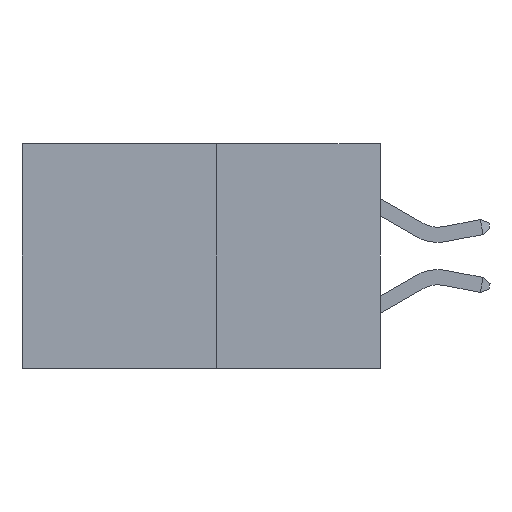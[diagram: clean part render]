
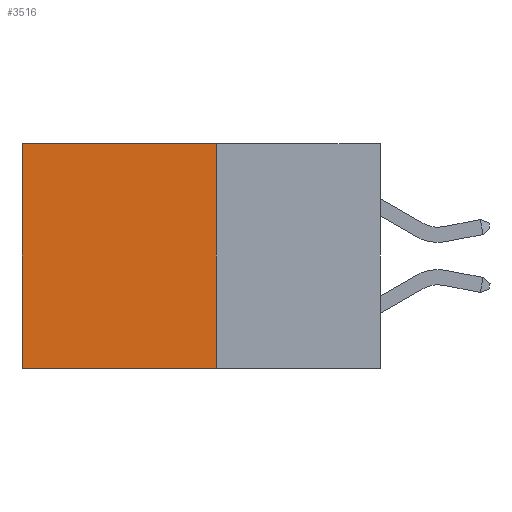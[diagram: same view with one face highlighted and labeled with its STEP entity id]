
A CAD part, left-side view. The second image highlights one B-rep face of the part: STEP entity #3516.
In plain terms, the highlighted planar face has unit normal (-1, 0, 0).
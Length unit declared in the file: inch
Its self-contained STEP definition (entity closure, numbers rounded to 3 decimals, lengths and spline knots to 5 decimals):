
#297 = AXIS2_PLACEMENT_3D ( 'NONE', #2258, #8689, #3286 ) ;
#330 = CARTESIAN_POINT ( 'NONE',  ( 0.277, 0.27, -0.37 ) ) ;
#347 = EDGE_LOOP ( 'NONE', ( #8659, #8934, #1839, #4963 ) ) ;
#608 = VECTOR ( 'NONE', #4120, 39.37008 ) ;
#1029 = CARTESIAN_POINT ( 'NONE',  ( 0.277, 0.27, -0.37 ) ) ;
#1249 = DIRECTION ( 'NONE',  ( 0., 0., -1. ) ) ;
#1362 = EDGE_CURVE ( 'NONE', #8119, #3547, #1634, .T. ) ;
#1634 = LINE ( 'NONE', #10024, #10639 ) ;
#1839 = ORIENTED_EDGE ( 'NONE', *, *, #2341, .F. ) ;
#2169 = EDGE_CURVE ( 'NONE', #3414, #7520, #5911, .T. ) ;
#2258 = CARTESIAN_POINT ( 'NONE',  ( 0.277, 0.27, -0.37 ) ) ;
#2341 = EDGE_CURVE ( 'NONE', #3414, #8119, #11596, .T. ) ;
#2356 = CARTESIAN_POINT ( 'NONE',  ( 0.277, 0.59, -0.37 ) ) ;
#2831 = EDGE_CURVE ( 'NONE', #7520, #3547, #8966, .T. ) ;
#3286 = DIRECTION ( 'NONE',  ( 0., 0., -1. ) ) ;
#3414 = VERTEX_POINT ( 'NONE', #7552 ) ;
#3516 = ADVANCED_FACE ( 'NONE', ( #6381 ), #11083, .F. ) ;
#3547 = VERTEX_POINT ( 'NONE', #2356 ) ;
#4120 = DIRECTION ( 'NONE',  ( 0., 1., 0. ) ) ;
#4290 = CARTESIAN_POINT ( 'NONE',  ( 0.277, 0.27, 0. ) ) ;
#4963 = ORIENTED_EDGE ( 'NONE', *, *, #2169, .T. ) ;
#5011 = VECTOR ( 'NONE', #1249, 39.37008 ) ;
#5911 = LINE ( 'NONE', #4290, #608 ) ;
#5962 = DIRECTION ( 'NONE',  ( 0., 1., 0. ) ) ;
#6196 = DIRECTION ( 'NONE',  ( 0., 0., -1. ) ) ;
#6381 = FACE_OUTER_BOUND ( 'NONE', #347, .T. ) ;
#6673 = VECTOR ( 'NONE', #6196, 39.37008 ) ;
#7260 = CARTESIAN_POINT ( 'NONE',  ( 0.277, 0.59, -0.37 ) ) ;
#7520 = VERTEX_POINT ( 'NONE', #10020 ) ;
#7552 = CARTESIAN_POINT ( 'NONE',  ( 0.277, 0.27, 0. ) ) ;
#8119 = VERTEX_POINT ( 'NONE', #330 ) ;
#8659 = ORIENTED_EDGE ( 'NONE', *, *, #2831, .T. ) ;
#8689 = DIRECTION ( 'NONE',  ( 1., 0., 0. ) ) ;
#8934 = ORIENTED_EDGE ( 'NONE', *, *, #1362, .F. ) ;
#8966 = LINE ( 'NONE', #7260, #6673 ) ;
#10020 = CARTESIAN_POINT ( 'NONE',  ( 0.277, 0.59, 0. ) ) ;
#10024 = CARTESIAN_POINT ( 'NONE',  ( 0.277, 0.27, -0.37 ) ) ;
#10639 = VECTOR ( 'NONE', #5962, 39.37008 ) ;
#11083 = PLANE ( 'NONE',  #297 ) ;
#11596 = LINE ( 'NONE', #1029, #5011 ) ;
